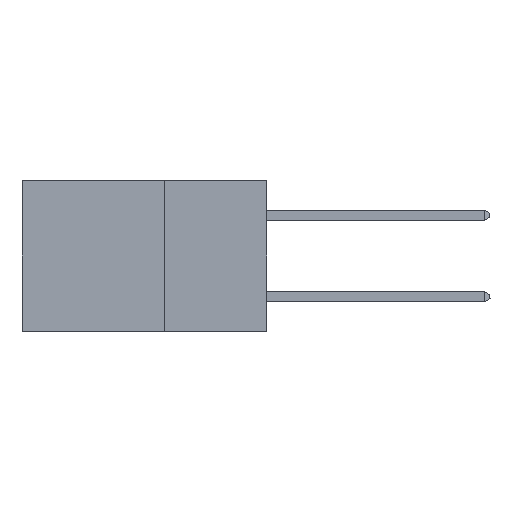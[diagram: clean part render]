
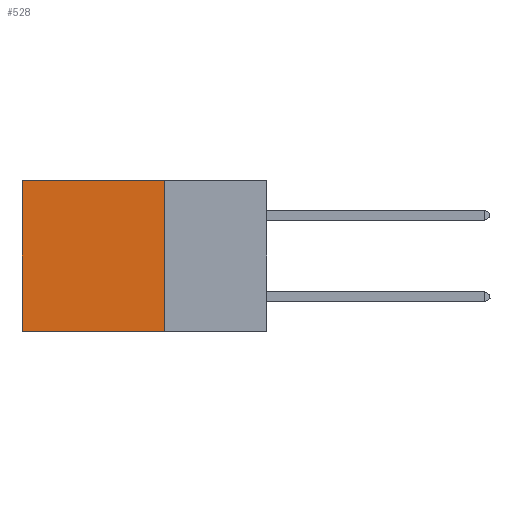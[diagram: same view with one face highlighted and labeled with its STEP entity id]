
A CAD part, left-side view. The second image highlights one B-rep face of the part: STEP entity #528.
In plain terms, the highlighted planar face has unit normal (-1, 0, 0).
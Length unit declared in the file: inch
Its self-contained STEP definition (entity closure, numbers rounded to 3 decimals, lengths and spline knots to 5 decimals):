
#314 = DIRECTION ( 'NONE',  ( 0., 1., 0. ) ) ;
#359 = EDGE_CURVE ( 'NONE', #5482, #8852, #8189, .T. ) ;
#528 = ADVANCED_FACE ( 'NONE', ( #12868 ), #631, .F. ) ;
#582 = EDGE_CURVE ( 'NONE', #8852, #9156, #12113, .T. ) ;
#631 = PLANE ( 'NONE',  #3990 ) ;
#1583 = VECTOR ( 'NONE', #14849, 39.37008 ) ;
#2307 = ORIENTED_EDGE ( 'NONE', *, *, #6142, .F. ) ;
#2905 = VECTOR ( 'NONE', #314, 39.37008 ) ;
#3885 = EDGE_LOOP ( 'NONE', ( #10807, #14863, #2307, #10534 ) ) ;
#3990 = AXIS2_PLACEMENT_3D ( 'NONE', #15573, #7921, #9419 ) ;
#5482 = VERTEX_POINT ( 'NONE', #6361 ) ;
#6071 = CARTESIAN_POINT ( 'NONE',  ( 0.2875, 0.25, -0.37 ) ) ;
#6142 = EDGE_CURVE ( 'NONE', #5482, #8957, #7246, .T. ) ;
#6180 = CARTESIAN_POINT ( 'NONE',  ( 0.2875, 0.25, 0. ) ) ;
#6361 = CARTESIAN_POINT ( 'NONE',  ( 0.2875, 0.25, 0. ) ) ;
#6516 = LINE ( 'NONE', #12141, #14862 ) ;
#7246 = LINE ( 'NONE', #6180, #1583 ) ;
#7921 = DIRECTION ( 'NONE',  ( 1., 0., 0. ) ) ;
#8160 = CARTESIAN_POINT ( 'NONE',  ( 0.2875, 0.6, -0.37 ) ) ;
#8189 = LINE ( 'NONE', #15246, #2905 ) ;
#8852 = VERTEX_POINT ( 'NONE', #15844 ) ;
#8957 = VERTEX_POINT ( 'NONE', #6071 ) ;
#9156 = VERTEX_POINT ( 'NONE', #8160 ) ;
#9257 = DIRECTION ( 'NONE',  ( 0., 0., -1. ) ) ;
#9419 = DIRECTION ( 'NONE',  ( 0., 0., -1. ) ) ;
#9749 = VECTOR ( 'NONE', #9257, 39.37008 ) ;
#10534 = ORIENTED_EDGE ( 'NONE', *, *, #359, .T. ) ;
#10535 = EDGE_CURVE ( 'NONE', #8957, #9156, #6516, .T. ) ;
#10807 = ORIENTED_EDGE ( 'NONE', *, *, #582, .T. ) ;
#12113 = LINE ( 'NONE', #14339, #9749 ) ;
#12141 = CARTESIAN_POINT ( 'NONE',  ( 0.2875, 0.25, -0.37 ) ) ;
#12195 = DIRECTION ( 'NONE',  ( 0., 1., 0. ) ) ;
#12868 = FACE_OUTER_BOUND ( 'NONE', #3885, .T. ) ;
#14339 = CARTESIAN_POINT ( 'NONE',  ( 0.2875, 0.6, 0. ) ) ;
#14849 = DIRECTION ( 'NONE',  ( 0., 0., -1. ) ) ;
#14862 = VECTOR ( 'NONE', #12195, 39.37008 ) ;
#14863 = ORIENTED_EDGE ( 'NONE', *, *, #10535, .F. ) ;
#15246 = CARTESIAN_POINT ( 'NONE',  ( 0.2875, 0.25, 0. ) ) ;
#15573 = CARTESIAN_POINT ( 'NONE',  ( 0.2875, 0.25, 0. ) ) ;
#15844 = CARTESIAN_POINT ( 'NONE',  ( 0.2875, 0.6, 0. ) ) ;
